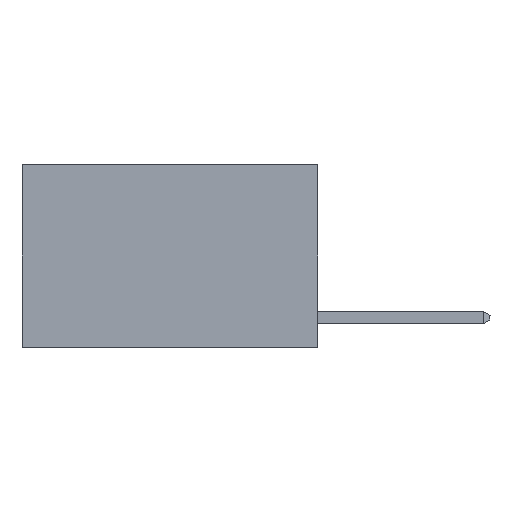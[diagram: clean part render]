
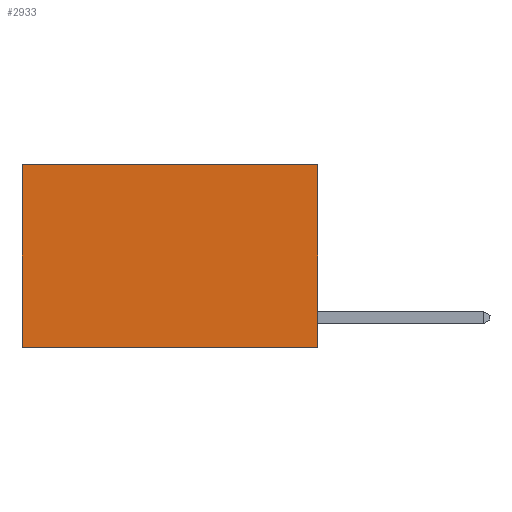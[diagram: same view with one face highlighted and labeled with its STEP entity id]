
A CAD part, left-side view. The second image highlights one B-rep face of the part: STEP entity #2933.
In plain terms, the highlighted planar face has unit normal (-1, 0, 0).
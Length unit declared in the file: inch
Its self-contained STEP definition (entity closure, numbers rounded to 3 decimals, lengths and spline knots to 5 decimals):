
#240 = CARTESIAN_POINT ( 'NONE',  ( 0.2625, 0., -0.37 ) ) ;
#561 = VERTEX_POINT ( 'NONE', #9991 ) ;
#1083 = EDGE_CURVE ( 'NONE', #561, #4084, #11544, .T. ) ;
#2087 = ORIENTED_EDGE ( 'NONE', *, *, #8749, .F. ) ;
#2105 = DIRECTION ( 'NONE',  ( 0., 1., 0. ) ) ;
#2325 = CARTESIAN_POINT ( 'NONE',  ( 0.2625, 0.6, 0. ) ) ;
#2334 = VECTOR ( 'NONE', #4499, 39.37008 ) ;
#2450 = DIRECTION ( 'NONE',  ( 0., 1., 0. ) ) ;
#2719 = CARTESIAN_POINT ( 'NONE',  ( 0.2625, 0., 0. ) ) ;
#2933 = ADVANCED_FACE ( 'NONE', ( #5075 ), #9323, .F. ) ;
#3747 = CARTESIAN_POINT ( 'NONE',  ( 0.2625, 0., 0. ) ) ;
#3789 = DIRECTION ( 'NONE',  ( 1., 0., 0. ) ) ;
#4084 = VERTEX_POINT ( 'NONE', #8002 ) ;
#4499 = DIRECTION ( 'NONE',  ( 0., 0., -1. ) ) ;
#5002 = CARTESIAN_POINT ( 'NONE',  ( 0.2625, 0.6, 0. ) ) ;
#5075 = FACE_OUTER_BOUND ( 'NONE', #13325, .T. ) ;
#5224 = LINE ( 'NONE', #2325, #2334 ) ;
#5635 = VECTOR ( 'NONE', #2450, 39.37008 ) ;
#5935 = VECTOR ( 'NONE', #9119, 39.37008 ) ;
#6031 = EDGE_CURVE ( 'NONE', #7425, #4084, #5224, .T. ) ;
#6248 = ORIENTED_EDGE ( 'NONE', *, *, #11600, .T. ) ;
#6355 = CARTESIAN_POINT ( 'NONE',  ( 0.2625, 0., 0. ) ) ;
#7425 = VERTEX_POINT ( 'NONE', #5002 ) ;
#7432 = AXIS2_PLACEMENT_3D ( 'NONE', #2719, #3789, #11649 ) ;
#7442 = VERTEX_POINT ( 'NONE', #3747 ) ;
#8002 = CARTESIAN_POINT ( 'NONE',  ( 0.2625, 0.6, -0.37 ) ) ;
#8613 = ORIENTED_EDGE ( 'NONE', *, *, #1083, .F. ) ;
#8749 = EDGE_CURVE ( 'NONE', #7442, #561, #13034, .T. ) ;
#9119 = DIRECTION ( 'NONE',  ( 0., 0., -1. ) ) ;
#9323 = PLANE ( 'NONE',  #7432 ) ;
#9442 = ORIENTED_EDGE ( 'NONE', *, *, #6031, .T. ) ;
#9991 = CARTESIAN_POINT ( 'NONE',  ( 0.2625, 0., -0.37 ) ) ;
#11449 = VECTOR ( 'NONE', #2105, 39.37008 ) ;
#11544 = LINE ( 'NONE', #240, #5635 ) ;
#11600 = EDGE_CURVE ( 'NONE', #7442, #7425, #11974, .T. ) ;
#11649 = DIRECTION ( 'NONE',  ( 0., 0., -1. ) ) ;
#11974 = LINE ( 'NONE', #13153, #11449 ) ;
#13034 = LINE ( 'NONE', #6355, #5935 ) ;
#13153 = CARTESIAN_POINT ( 'NONE',  ( 0.2625, 0., 0. ) ) ;
#13325 = EDGE_LOOP ( 'NONE', ( #9442, #8613, #2087, #6248 ) ) ;
